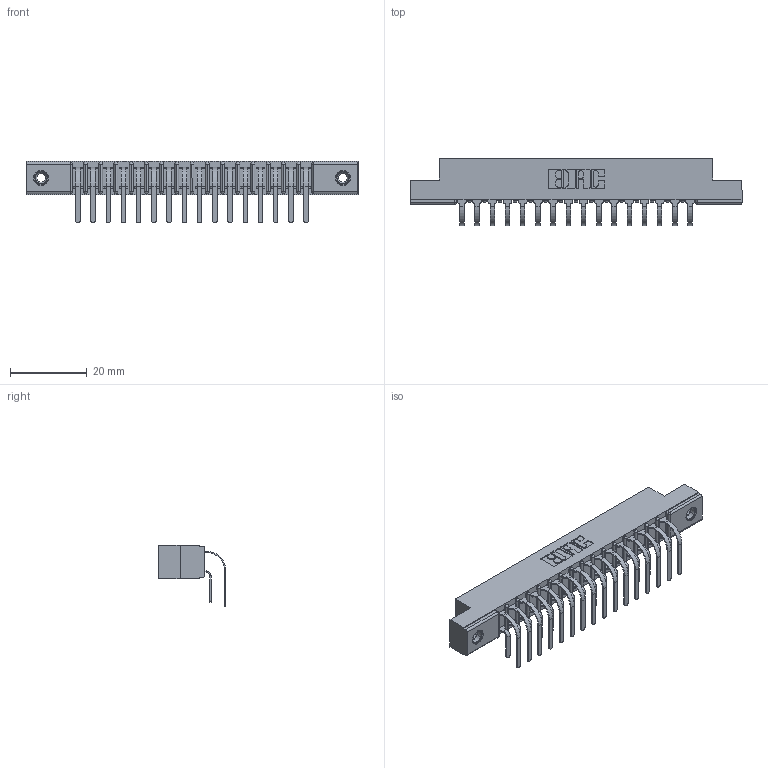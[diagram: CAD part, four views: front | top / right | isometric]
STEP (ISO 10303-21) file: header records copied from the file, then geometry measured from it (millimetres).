
FILE_DESCRIPTION (( 'STEP AP203' ), '1' );
FILE_NAME ('357-032-559-208.STEP', '2022-07-08T23:45:10', ( '' ), ( '' ), 'SwSTEP 2.0', 'SolidWorks 2020', '' );
FILE_SCHEMA (( 'CONFIG_CONTROL_DESIGN' ));
Length unit declared in the file: inch
Products named in the file (5): 307 Part_.156 Dia Mounting Holes; 345-250-001_345-250-003-102; 307-290-001_559 - 2 (Single); 357-032-559-208; 307-290-001_558 559 - 1 (Single)
Assembly tree (35 placements, depth 2):
  357-032-559-208
    307 Part_.156 Dia Mounting Holes
    307-290-001_558 559 - 1 (Single)  x16
    307-290-001_559 - 2 (Single)  x16
    345-250-001_345-250-003-102  x2
Bounding box: 86.41 x 17.51 x 16.08 mm (x, y, z)
Volume: 5766.7 mm3; surface area: 10563.7 mm2
Topology: 35 solids, 35 shells, 1795 faces, 5003 edges, 3238 vertices
Faces by surface type: plane 1158, cylinder 587, sphere 34, cone 12, torus 4
Entity records: 20066 total; most frequent: CARTESIAN_POINT 3277, ORIENTED_EDGE 3238, DIRECTION 3229, EDGE_CURVE 1619, LINE 1229, VECTOR 1229, VERTEX_POINT 1048, AXIS2_PLACEMENT_3D 1000
